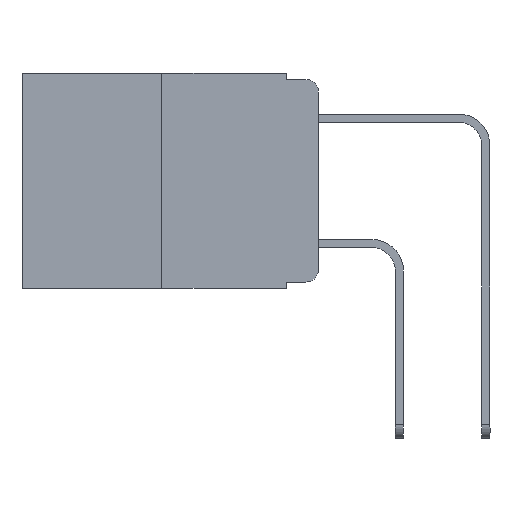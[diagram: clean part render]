
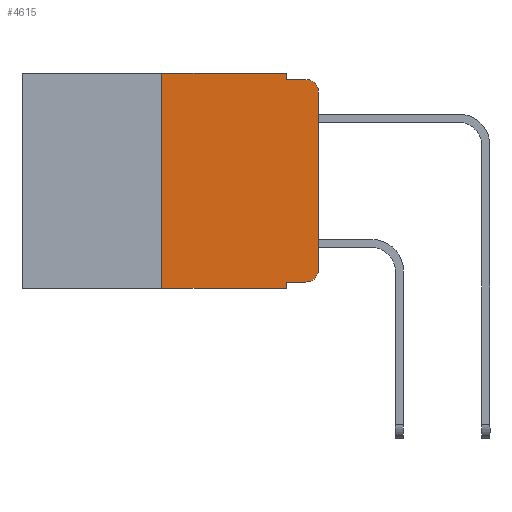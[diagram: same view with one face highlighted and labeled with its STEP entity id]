
A CAD part, left-side view. The second image highlights one B-rep face of the part: STEP entity #4615.
In plain terms, the highlighted planar face has unit normal (-1, 0, 0).
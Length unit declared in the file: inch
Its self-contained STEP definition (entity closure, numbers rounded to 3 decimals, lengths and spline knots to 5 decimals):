
#70 = CARTESIAN_POINT ( 'NONE',  ( 0., 0., -0.03 ) ) ;
#151 = DIRECTION ( 'NONE',  ( 0., 0., -1. ) ) ;
#323 = ORIENTED_EDGE ( 'NONE', *, *, #13538, .F. ) ;
#952 = VERTEX_POINT ( 'NONE', #11935 ) ;
#1342 = CARTESIAN_POINT ( 'NONE',  ( 0., 0.02, -0.03 ) ) ;
#1364 = CARTESIAN_POINT ( 'NONE',  ( 0., 0.25, -0.343 ) ) ;
#1621 = AXIS2_PLACEMENT_3D ( 'NONE', #1342, #16207, #151 ) ;
#1882 = DIRECTION ( 'NONE',  ( 0., 0., -1. ) ) ;
#2223 = VERTEX_POINT ( 'NONE', #11560 ) ;
#2358 = CARTESIAN_POINT ( 'NONE',  ( 0., 0.051, -0.333 ) ) ;
#2860 = VECTOR ( 'NONE', #8573, 39.37008 ) ;
#2890 = VERTEX_POINT ( 'NONE', #13773 ) ;
#2988 = EDGE_CURVE ( 'NONE', #13738, #6979, #5068, .T. ) ;
#3144 = VERTEX_POINT ( 'NONE', #7225 ) ;
#3551 = EDGE_LOOP ( 'NONE', ( #6506, #16317, #8285, #14889, #14743, #323, #11742, #11065, #8591, #7252 ) ) ;
#3588 = CARTESIAN_POINT ( 'NONE',  ( 0., 0.25, 0. ) ) ;
#4615 = ADVANCED_FACE ( 'NONE', ( #16060 ), #12181, .F. ) ;
#4861 = LINE ( 'NONE', #8477, #2860 ) ;
#5068 = CIRCLE ( 'NONE', #9369, 0.02 ) ;
#5089 = EDGE_CURVE ( 'NONE', #2223, #952, #15873, .T. ) ;
#5215 = DIRECTION ( 'NONE',  ( 0., -1., 0. ) ) ;
#5758 = DIRECTION ( 'NONE',  ( 0., 0., 1. ) ) ;
#5981 = VERTEX_POINT ( 'NONE', #15913 ) ;
#6057 = CARTESIAN_POINT ( 'NONE',  ( 0., 0.473, 0. ) ) ;
#6506 = ORIENTED_EDGE ( 'NONE', *, *, #15606, .T. ) ;
#6637 = DIRECTION ( 'NONE',  ( 0., 0., -1. ) ) ;
#6738 = AXIS2_PLACEMENT_3D ( 'NONE', #6057, #13371, #1882 ) ;
#6979 = VERTEX_POINT ( 'NONE', #7549 ) ;
#7225 = CARTESIAN_POINT ( 'NONE',  ( 0., 0.051, -0.343 ) ) ;
#7252 = ORIENTED_EDGE ( 'NONE', *, *, #2988, .T. ) ;
#7342 = CARTESIAN_POINT ( 'NONE',  ( 0., 0.473, -0.343 ) ) ;
#7365 = CARTESIAN_POINT ( 'NONE',  ( 0., 0., 0. ) ) ;
#7520 = LINE ( 'NONE', #16485, #13950 ) ;
#7549 = CARTESIAN_POINT ( 'NONE',  ( 0., 0., -0.313 ) ) ;
#7698 = LINE ( 'NONE', #8787, #7757 ) ;
#7757 = VECTOR ( 'NONE', #11229, 39.37008 ) ;
#8056 = CARTESIAN_POINT ( 'NONE',  ( 0., 0.02, -0.333 ) ) ;
#8285 = ORIENTED_EDGE ( 'NONE', *, *, #5089, .F. ) ;
#8477 = CARTESIAN_POINT ( 'NONE',  ( 0., 0.473, 0. ) ) ;
#8573 = DIRECTION ( 'NONE',  ( 0., -1., 0. ) ) ;
#8591 = ORIENTED_EDGE ( 'NONE', *, *, #11800, .T. ) ;
#8662 = VECTOR ( 'NONE', #9581, 39.37008 ) ;
#8673 = DIRECTION ( 'NONE',  ( 0., -1., 0. ) ) ;
#8787 = CARTESIAN_POINT ( 'NONE',  ( 0., 0.051, 0. ) ) ;
#9068 = CARTESIAN_POINT ( 'NONE',  ( 0., 0.02, -0.313 ) ) ;
#9164 = DIRECTION ( 'NONE',  ( -1., 0., 0. ) ) ;
#9369 = AXIS2_PLACEMENT_3D ( 'NONE', #9068, #9164, #6637 ) ;
#9581 = DIRECTION ( 'NONE',  ( 0., -1., 0. ) ) ;
#10184 = LINE ( 'NONE', #2358, #15551 ) ;
#10731 = VERTEX_POINT ( 'NONE', #12110 ) ;
#11065 = ORIENTED_EDGE ( 'NONE', *, *, #12476, .F. ) ;
#11114 = LINE ( 'NONE', #7342, #12500 ) ;
#11224 = VECTOR ( 'NONE', #11644, 39.37008 ) ;
#11229 = DIRECTION ( 'NONE',  ( 0., 0., -1. ) ) ;
#11356 = EDGE_CURVE ( 'NONE', #16314, #952, #14458, .T. ) ;
#11560 = CARTESIAN_POINT ( 'NONE',  ( 0., 0.051, -0.01 ) ) ;
#11644 = DIRECTION ( 'NONE',  ( 0., 0., 1. ) ) ;
#11742 = ORIENTED_EDGE ( 'NONE', *, *, #12953, .T. ) ;
#11800 = EDGE_CURVE ( 'NONE', #10731, #13738, #10184, .T. ) ;
#11935 = CARTESIAN_POINT ( 'NONE',  ( 0., 0.02, -0.01 ) ) ;
#12110 = CARTESIAN_POINT ( 'NONE',  ( 0., 0.051, -0.333 ) ) ;
#12161 = CARTESIAN_POINT ( 'NONE',  ( 0., 0.051, -0.01 ) ) ;
#12181 = PLANE ( 'NONE',  #6738 ) ;
#12476 = EDGE_CURVE ( 'NONE', #10731, #3144, #7520, .T. ) ;
#12500 = VECTOR ( 'NONE', #8673, 39.37008 ) ;
#12953 = EDGE_CURVE ( 'NONE', #14791, #3144, #11114, .T. ) ;
#13335 = EDGE_CURVE ( 'NONE', #5981, #2890, #4861, .T. ) ;
#13371 = DIRECTION ( 'NONE',  ( 1., 0., 0. ) ) ;
#13538 = EDGE_CURVE ( 'NONE', #14791, #5981, #14009, .T. ) ;
#13649 = LINE ( 'NONE', #7365, #14695 ) ;
#13738 = VERTEX_POINT ( 'NONE', #8056 ) ;
#13773 = CARTESIAN_POINT ( 'NONE',  ( 0., 0.051, 0. ) ) ;
#13883 = EDGE_CURVE ( 'NONE', #2890, #2223, #7698, .T. ) ;
#13950 = VECTOR ( 'NONE', #15130, 39.37008 ) ;
#14009 = LINE ( 'NONE', #3588, #11224 ) ;
#14458 = CIRCLE ( 'NONE', #1621, 0.02 ) ;
#14695 = VECTOR ( 'NONE', #5758, 39.37008 ) ;
#14743 = ORIENTED_EDGE ( 'NONE', *, *, #13335, .F. ) ;
#14791 = VERTEX_POINT ( 'NONE', #1364 ) ;
#14889 = ORIENTED_EDGE ( 'NONE', *, *, #13883, .F. ) ;
#15130 = DIRECTION ( 'NONE',  ( 0., 0., -1. ) ) ;
#15551 = VECTOR ( 'NONE', #5215, 39.37008 ) ;
#15606 = EDGE_CURVE ( 'NONE', #6979, #16314, #13649, .T. ) ;
#15873 = LINE ( 'NONE', #12161, #8662 ) ;
#15913 = CARTESIAN_POINT ( 'NONE',  ( 0., 0.25, 0. ) ) ;
#16060 = FACE_OUTER_BOUND ( 'NONE', #3551, .T. ) ;
#16207 = DIRECTION ( 'NONE',  ( -1., 0., 0. ) ) ;
#16314 = VERTEX_POINT ( 'NONE', #70 ) ;
#16317 = ORIENTED_EDGE ( 'NONE', *, *, #11356, .T. ) ;
#16485 = CARTESIAN_POINT ( 'NONE',  ( 0., 0.051, 0. ) ) ;
